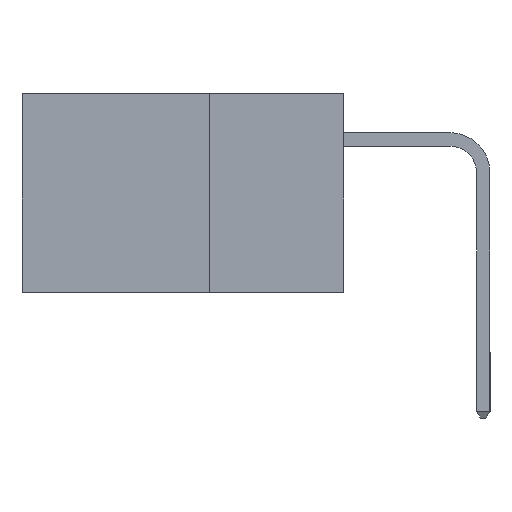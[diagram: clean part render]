
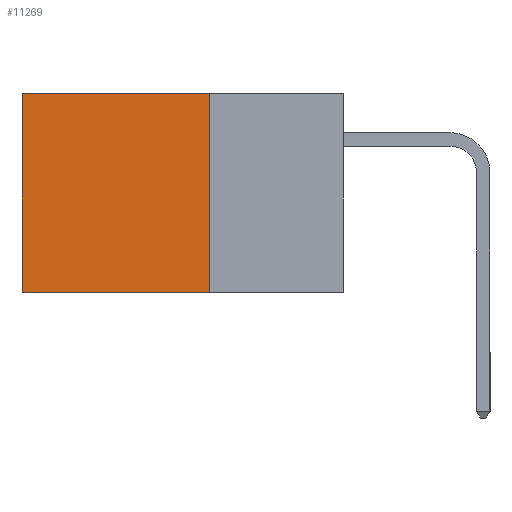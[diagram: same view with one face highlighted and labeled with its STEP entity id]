
A CAD part, left-side view. The second image highlights one B-rep face of the part: STEP entity #11269.
In plain terms, the highlighted planar face has unit normal (-1, 0, 0).
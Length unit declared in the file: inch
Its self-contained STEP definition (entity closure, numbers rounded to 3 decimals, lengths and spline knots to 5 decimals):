
#1156 = VECTOR ( 'NONE', #5126, 39.37008 ) ;
#1449 = FACE_OUTER_BOUND ( 'NONE', #16535, .T. ) ;
#1942 = LINE ( 'NONE', #9512, #5842 ) ;
#2325 = CARTESIAN_POINT ( 'NONE',  ( 0.298, 0.6, -0.37 ) ) ;
#3753 = LINE ( 'NONE', #12471, #18011 ) ;
#4675 = DIRECTION ( 'NONE',  ( 0., 1., 0. ) ) ;
#5060 = EDGE_CURVE ( 'NONE', #14699, #11807, #1942, .T. ) ;
#5126 = DIRECTION ( 'NONE',  ( 0., 0., -1. ) ) ;
#5426 = CARTESIAN_POINT ( 'NONE',  ( 0.298, 0.25, 0. ) ) ;
#5780 = LINE ( 'NONE', #18762, #1156 ) ;
#5842 = VECTOR ( 'NONE', #12498, 39.37008 ) ;
#5894 = DIRECTION ( 'NONE',  ( 0., 0., -1. ) ) ;
#6350 = EDGE_CURVE ( 'NONE', #10642, #14699, #5780, .T. ) ;
#6539 = PLANE ( 'NONE',  #18579 ) ;
#7012 = CARTESIAN_POINT ( 'NONE',  ( 0.298, 0.6, 0. ) ) ;
#9512 = CARTESIAN_POINT ( 'NONE',  ( 0.298, 0.25, -0.37 ) ) ;
#9976 = DIRECTION ( 'NONE',  ( 1., 0., 0. ) ) ;
#9991 = ORIENTED_EDGE ( 'NONE', *, *, #5060, .F. ) ;
#10099 = LINE ( 'NONE', #15211, #18442 ) ;
#10210 = ORIENTED_EDGE ( 'NONE', *, *, #15299, .T. ) ;
#10642 = VERTEX_POINT ( 'NONE', #5426 ) ;
#11269 = ADVANCED_FACE ( 'NONE', ( #1449 ), #6539, .F. ) ;
#11807 = VERTEX_POINT ( 'NONE', #2325 ) ;
#12471 = CARTESIAN_POINT ( 'NONE',  ( 0.298, 0.25, 0. ) ) ;
#12498 = DIRECTION ( 'NONE',  ( 0., 1., 0. ) ) ;
#12987 = EDGE_CURVE ( 'NONE', #10642, #13298, #3753, .T. ) ;
#13298 = VERTEX_POINT ( 'NONE', #7012 ) ;
#14195 = CARTESIAN_POINT ( 'NONE',  ( 0.298, 0.25, -0.37 ) ) ;
#14699 = VERTEX_POINT ( 'NONE', #14195 ) ;
#15211 = CARTESIAN_POINT ( 'NONE',  ( 0.298, 0.6, 0. ) ) ;
#15299 = EDGE_CURVE ( 'NONE', #13298, #11807, #10099, .T. ) ;
#16123 = ORIENTED_EDGE ( 'NONE', *, *, #6350, .F. ) ;
#16535 = EDGE_LOOP ( 'NONE', ( #10210, #9991, #16123, #17211 ) ) ;
#17211 = ORIENTED_EDGE ( 'NONE', *, *, #12987, .T. ) ;
#18011 = VECTOR ( 'NONE', #4675, 39.37008 ) ;
#18442 = VECTOR ( 'NONE', #5894, 39.37008 ) ;
#18579 = AXIS2_PLACEMENT_3D ( 'NONE', #19349, #9976, #19207 ) ;
#18762 = CARTESIAN_POINT ( 'NONE',  ( 0.298, 0.25, 0. ) ) ;
#19207 = DIRECTION ( 'NONE',  ( 0., 0., -1. ) ) ;
#19349 = CARTESIAN_POINT ( 'NONE',  ( 0.298, 0.25, 0. ) ) ;
